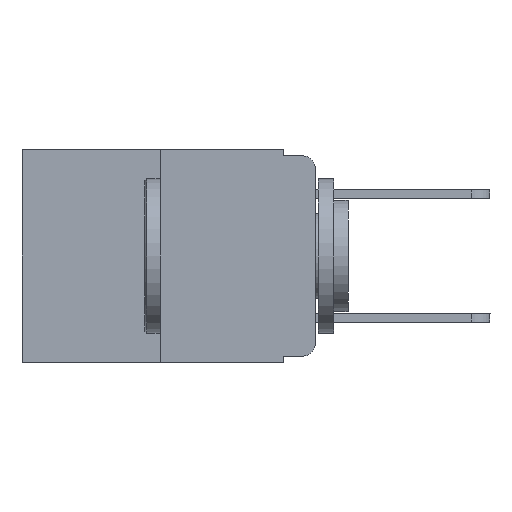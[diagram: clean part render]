
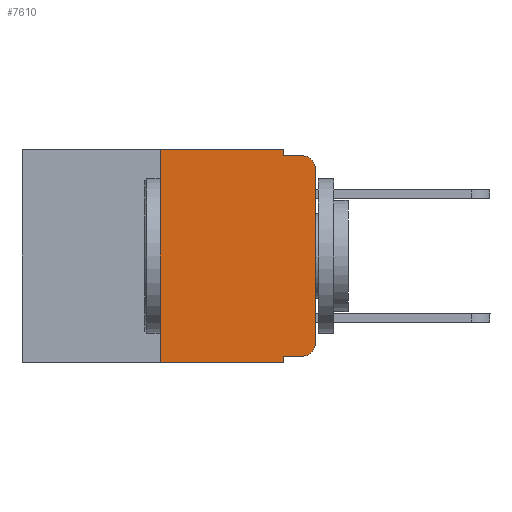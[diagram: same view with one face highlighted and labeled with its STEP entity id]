
A CAD part, left-side view. The second image highlights one B-rep face of the part: STEP entity #7610.
In plain terms, the highlighted planar face has unit normal (-1, 0, 0).
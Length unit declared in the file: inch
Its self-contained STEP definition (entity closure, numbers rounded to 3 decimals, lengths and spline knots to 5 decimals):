
#13 = VECTOR ( 'NONE', #3254, 39.37008 ) ;
#82 = AXIS2_PLACEMENT_3D ( 'NONE', #6932, #2071, #8261 ) ;
#329 = EDGE_CURVE ( 'NONE', #3363, #4260, #11998, .T. ) ;
#789 = DIRECTION ( 'NONE',  ( 0., -1., 0. ) ) ;
#957 = ORIENTED_EDGE ( 'NONE', *, *, #14550, .F. ) ;
#1031 = DIRECTION ( 'NONE',  ( 0., 0., -1. ) ) ;
#1145 = CARTESIAN_POINT ( 'NONE',  ( 0., 0.051, -0.333 ) ) ;
#1305 = CARTESIAN_POINT ( 'NONE',  ( 0., 0.051, -0.01 ) ) ;
#1337 = VECTOR ( 'NONE', #2305, 39.37008 ) ;
#1603 = VECTOR ( 'NONE', #1031, 39.37008 ) ;
#1641 = VECTOR ( 'NONE', #2199, 39.37008 ) ;
#1730 = DIRECTION ( 'NONE',  ( 0., 0., 1. ) ) ;
#1731 = PLANE ( 'NONE',  #2946 ) ;
#2071 = DIRECTION ( 'NONE',  ( -1., 0., 0. ) ) ;
#2199 = DIRECTION ( 'NONE',  ( 0., -1., 0. ) ) ;
#2305 = DIRECTION ( 'NONE',  ( 0., -1., 0. ) ) ;
#2318 = VERTEX_POINT ( 'NONE', #15734 ) ;
#2355 = DIRECTION ( 'NONE',  ( 0., -1., 0. ) ) ;
#2376 = VECTOR ( 'NONE', #1730, 39.37008 ) ;
#2539 = DIRECTION ( 'NONE',  ( -1., 0., 0. ) ) ;
#2946 = AXIS2_PLACEMENT_3D ( 'NONE', #2980, #15551, #11699 ) ;
#2980 = CARTESIAN_POINT ( 'NONE',  ( 0., 0.473, 0. ) ) ;
#3158 = EDGE_CURVE ( 'NONE', #5438, #12234, #4152, .T. ) ;
#3254 = DIRECTION ( 'NONE',  ( 0., 0., 1. ) ) ;
#3315 = VERTEX_POINT ( 'NONE', #12994 ) ;
#3363 = VERTEX_POINT ( 'NONE', #1305 ) ;
#3424 = CARTESIAN_POINT ( 'NONE',  ( 0., 0.473, 0. ) ) ;
#3751 = CIRCLE ( 'NONE', #12318, 0.02 ) ;
#3846 = VERTEX_POINT ( 'NONE', #7544 ) ;
#3869 = EDGE_CURVE ( 'NONE', #3846, #10216, #3751, .T. ) ;
#4152 = LINE ( 'NONE', #14568, #12185 ) ;
#4260 = VERTEX_POINT ( 'NONE', #13515 ) ;
#4585 = EDGE_CURVE ( 'NONE', #2318, #12234, #11733, .T. ) ;
#4770 = CARTESIAN_POINT ( 'NONE',  ( 0., 0., -0.03 ) ) ;
#4775 = CIRCLE ( 'NONE', #82, 0.02 ) ;
#4810 = EDGE_CURVE ( 'NONE', #5438, #12701, #11929, .T. ) ;
#5122 = LINE ( 'NONE', #13104, #7686 ) ;
#5209 = VECTOR ( 'NONE', #2355, 39.37008 ) ;
#5438 = VERTEX_POINT ( 'NONE', #6225 ) ;
#5769 = ORIENTED_EDGE ( 'NONE', *, *, #3158, .T. ) ;
#5780 = EDGE_CURVE ( 'NONE', #10216, #7151, #11519, .T. ) ;
#6020 = CARTESIAN_POINT ( 'NONE',  ( 0., 0.051, 0. ) ) ;
#6225 = CARTESIAN_POINT ( 'NONE',  ( 0., 0.25, -0.343 ) ) ;
#6556 = LINE ( 'NONE', #1145, #5209 ) ;
#6932 = CARTESIAN_POINT ( 'NONE',  ( 0., 0.02, -0.03 ) ) ;
#7107 = EDGE_CURVE ( 'NONE', #12701, #3315, #7962, .T. ) ;
#7151 = VERTEX_POINT ( 'NONE', #4770 ) ;
#7201 = EDGE_CURVE ( 'NONE', #2318, #3846, #6556, .T. ) ;
#7544 = CARTESIAN_POINT ( 'NONE',  ( 0., 0.02, -0.333 ) ) ;
#7610 = ADVANCED_FACE ( 'NONE', ( #11854 ), #1731, .F. ) ;
#7686 = VECTOR ( 'NONE', #13048, 39.37008 ) ;
#7962 = LINE ( 'NONE', #3424, #1337 ) ;
#8261 = DIRECTION ( 'NONE',  ( 0., 0., -1. ) ) ;
#8401 = CARTESIAN_POINT ( 'NONE',  ( 0., 0.051, -0.01 ) ) ;
#8664 = CARTESIAN_POINT ( 'NONE',  ( 0., 0.25, 0. ) ) ;
#8842 = CARTESIAN_POINT ( 'NONE',  ( 0., 0.051, -0.343 ) ) ;
#9347 = ORIENTED_EDGE ( 'NONE', *, *, #7201, .T. ) ;
#9909 = ORIENTED_EDGE ( 'NONE', *, *, #3869, .T. ) ;
#10216 = VERTEX_POINT ( 'NONE', #14157 ) ;
#10315 = ORIENTED_EDGE ( 'NONE', *, *, #4585, .F. ) ;
#11081 = ORIENTED_EDGE ( 'NONE', *, *, #7107, .F. ) ;
#11200 = CARTESIAN_POINT ( 'NONE',  ( 0., 0.02, -0.313 ) ) ;
#11257 = ORIENTED_EDGE ( 'NONE', *, *, #329, .F. ) ;
#11258 = DIRECTION ( 'NONE',  ( 0., 0., -1. ) ) ;
#11519 = LINE ( 'NONE', #14538, #13 ) ;
#11699 = DIRECTION ( 'NONE',  ( 0., 0., -1. ) ) ;
#11733 = LINE ( 'NONE', #6020, #1603 ) ;
#11854 = FACE_OUTER_BOUND ( 'NONE', #15530, .T. ) ;
#11929 = LINE ( 'NONE', #14350, #2376 ) ;
#11998 = LINE ( 'NONE', #8401, #1641 ) ;
#12185 = VECTOR ( 'NONE', #789, 39.37008 ) ;
#12234 = VERTEX_POINT ( 'NONE', #8842 ) ;
#12318 = AXIS2_PLACEMENT_3D ( 'NONE', #11200, #2539, #11258 ) ;
#12701 = VERTEX_POINT ( 'NONE', #8664 ) ;
#12994 = CARTESIAN_POINT ( 'NONE',  ( 0., 0.051, 0. ) ) ;
#13048 = DIRECTION ( 'NONE',  ( 0., 0., -1. ) ) ;
#13104 = CARTESIAN_POINT ( 'NONE',  ( 0., 0.051, 0. ) ) ;
#13515 = CARTESIAN_POINT ( 'NONE',  ( 0., 0.02, -0.01 ) ) ;
#13669 = EDGE_CURVE ( 'NONE', #7151, #4260, #4775, .T. ) ;
#14157 = CARTESIAN_POINT ( 'NONE',  ( 0., 0., -0.313 ) ) ;
#14350 = CARTESIAN_POINT ( 'NONE',  ( 0., 0.25, 0. ) ) ;
#14538 = CARTESIAN_POINT ( 'NONE',  ( 0., 0., 0. ) ) ;
#14550 = EDGE_CURVE ( 'NONE', #3315, #3363, #5122, .T. ) ;
#14568 = CARTESIAN_POINT ( 'NONE',  ( 0., 0.473, -0.343 ) ) ;
#14671 = ORIENTED_EDGE ( 'NONE', *, *, #4810, .F. ) ;
#15530 = EDGE_LOOP ( 'NONE', ( #16036, #15856, #11257, #957, #11081, #14671, #5769, #10315, #9347, #9909 ) ) ;
#15551 = DIRECTION ( 'NONE',  ( 1., 0., 0. ) ) ;
#15734 = CARTESIAN_POINT ( 'NONE',  ( 0., 0.051, -0.333 ) ) ;
#15856 = ORIENTED_EDGE ( 'NONE', *, *, #13669, .T. ) ;
#16036 = ORIENTED_EDGE ( 'NONE', *, *, #5780, .T. ) ;
